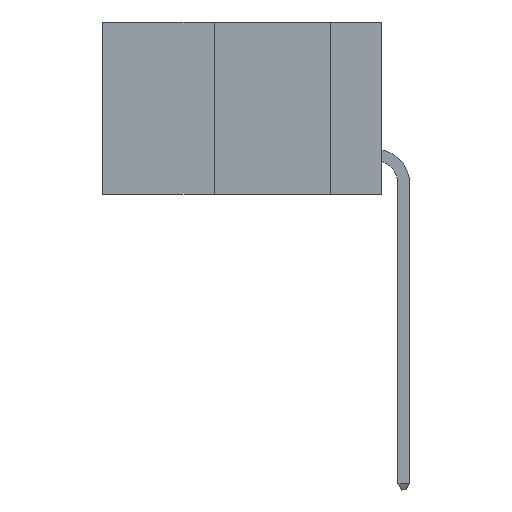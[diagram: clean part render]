
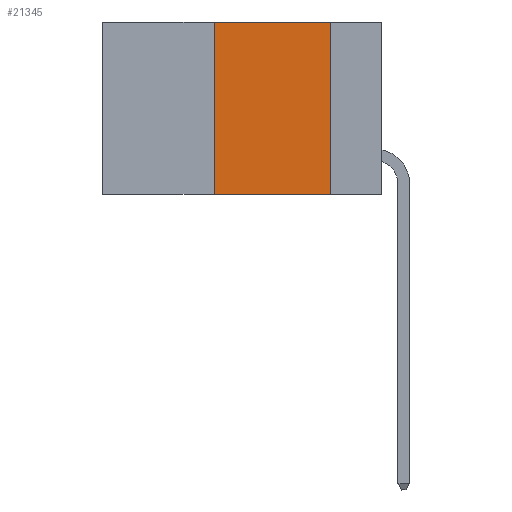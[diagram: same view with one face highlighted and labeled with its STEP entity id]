
A CAD part, left-side view. The second image highlights one B-rep face of the part: STEP entity #21345.
In plain terms, the highlighted planar face has unit normal (-1, 0, 0).
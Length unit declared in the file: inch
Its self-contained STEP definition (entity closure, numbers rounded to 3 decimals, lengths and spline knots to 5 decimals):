
#53 = EDGE_LOOP ( 'NONE', ( #22078, #18372, #20820, #8570 ) ) ;
#964 = EDGE_CURVE ( 'NONE', #20922, #5994, #17781, .T. ) ;
#1718 = CARTESIAN_POINT ( 'NONE',  ( 0., 0.6, -0.37 ) ) ;
#1894 = VERTEX_POINT ( 'NONE', #5210 ) ;
#1896 = DIRECTION ( 'NONE',  ( 0., 0., -1. ) ) ;
#1982 = EDGE_CURVE ( 'NONE', #20922, #1894, #14771, .T. ) ;
#3946 = DIRECTION ( 'NONE',  ( 0., 0., -1. ) ) ;
#3954 = VECTOR ( 'NONE', #10874, 39.37008 ) ;
#3974 = CARTESIAN_POINT ( 'NONE',  ( 0., 0.6, 0. ) ) ;
#5210 = CARTESIAN_POINT ( 'NONE',  ( 0., 0.11, -0.37 ) ) ;
#5849 = CARTESIAN_POINT ( 'NONE',  ( 0., 0.11, 0. ) ) ;
#5994 = VERTEX_POINT ( 'NONE', #13675 ) ;
#6571 = CARTESIAN_POINT ( 'NONE',  ( 0., 0.36, 0. ) ) ;
#8570 = ORIENTED_EDGE ( 'NONE', *, *, #1982, .T. ) ;
#8967 = LINE ( 'NONE', #14478, #3954 ) ;
#10260 = DIRECTION ( 'NONE',  ( 0., 0., 1. ) ) ;
#10874 = DIRECTION ( 'NONE',  ( 0., -1., 0. ) ) ;
#11155 = CARTESIAN_POINT ( 'NONE',  ( 0., 0.36, -0.37 ) ) ;
#11196 = DIRECTION ( 'NONE',  ( 0., -1., 0. ) ) ;
#11376 = PLANE ( 'NONE',  #24069 ) ;
#13675 = CARTESIAN_POINT ( 'NONE',  ( 0., 0.36, 0. ) ) ;
#13932 = LINE ( 'NONE', #5849, #14519 ) ;
#14478 = CARTESIAN_POINT ( 'NONE',  ( 0., 0.6, 0. ) ) ;
#14519 = VECTOR ( 'NONE', #3946, 39.37008 ) ;
#14771 = LINE ( 'NONE', #1718, #23041 ) ;
#16005 = VECTOR ( 'NONE', #10260, 39.37008 ) ;
#17030 = FACE_OUTER_BOUND ( 'NONE', #53, .T. ) ;
#17401 = VERTEX_POINT ( 'NONE', #21761 ) ;
#17493 = EDGE_CURVE ( 'NONE', #5994, #17401, #8967, .T. ) ;
#17781 = LINE ( 'NONE', #6571, #16005 ) ;
#17825 = EDGE_CURVE ( 'NONE', #17401, #1894, #13932, .T. ) ;
#18372 = ORIENTED_EDGE ( 'NONE', *, *, #17493, .F. ) ;
#19046 = DIRECTION ( 'NONE',  ( 1., 0., 0. ) ) ;
#20820 = ORIENTED_EDGE ( 'NONE', *, *, #964, .F. ) ;
#20922 = VERTEX_POINT ( 'NONE', #11155 ) ;
#21345 = ADVANCED_FACE ( 'NONE', ( #17030 ), #11376, .F. ) ;
#21761 = CARTESIAN_POINT ( 'NONE',  ( 0., 0.11, 0. ) ) ;
#22078 = ORIENTED_EDGE ( 'NONE', *, *, #17825, .F. ) ;
#23041 = VECTOR ( 'NONE', #11196, 39.37008 ) ;
#24069 = AXIS2_PLACEMENT_3D ( 'NONE', #3974, #19046, #1896 ) ;
